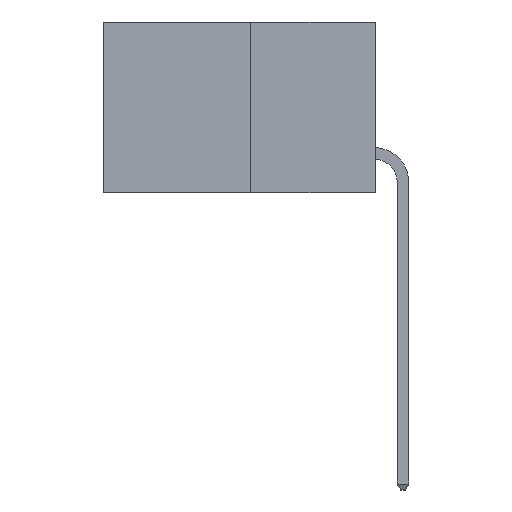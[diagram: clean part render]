
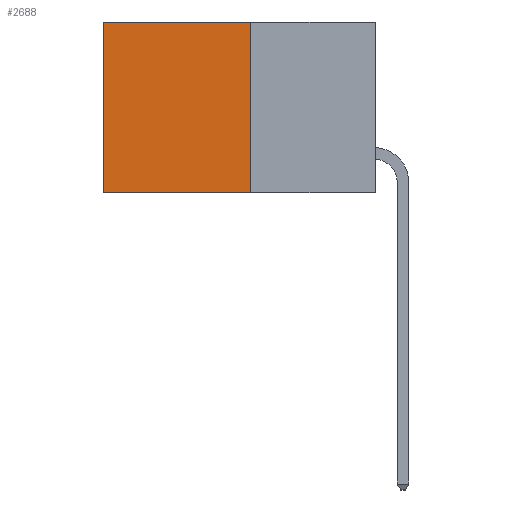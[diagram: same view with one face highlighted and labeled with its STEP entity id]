
A CAD part, left-side view. The second image highlights one B-rep face of the part: STEP entity #2688.
In plain terms, the highlighted planar face has unit normal (-1, 0, 0).
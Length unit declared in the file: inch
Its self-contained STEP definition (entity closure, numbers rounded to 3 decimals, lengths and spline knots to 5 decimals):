
#168 = ORIENTED_EDGE ( 'NONE', *, *, #8321, .T. ) ;
#222 = ORIENTED_EDGE ( 'NONE', *, *, #2465, .F. ) ;
#469 = VERTEX_POINT ( 'NONE', #6813 ) ;
#505 = DIRECTION ( 'NONE',  ( 0., 1., 0. ) ) ;
#796 = DIRECTION ( 'NONE',  ( 0., 1., 0. ) ) ;
#940 = ORIENTED_EDGE ( 'NONE', *, *, #5867, .F. ) ;
#1009 = ORIENTED_EDGE ( 'NONE', *, *, #9448, .T. ) ;
#1093 = VERTEX_POINT ( 'NONE', #1845 ) ;
#1612 = AXIS2_PLACEMENT_3D ( 'NONE', #3009, #3651, #3629 ) ;
#1795 = LINE ( 'NONE', #5422, #3863 ) ;
#1845 = CARTESIAN_POINT ( 'NONE',  ( 0.277, 0.27, -0.37 ) ) ;
#2310 = EDGE_LOOP ( 'NONE', ( #168, #222, #940, #1009 ) ) ;
#2465 = EDGE_CURVE ( 'NONE', #1093, #5009, #3487, .T. ) ;
#2473 = LINE ( 'NONE', #3248, #8045 ) ;
#2688 = ADVANCED_FACE ( 'NONE', ( #8887 ), #2807, .F. ) ;
#2807 = PLANE ( 'NONE',  #1612 ) ;
#3009 = CARTESIAN_POINT ( 'NONE',  ( 0.277, 0.27, -0.37 ) ) ;
#3248 = CARTESIAN_POINT ( 'NONE',  ( 0.277, 0.59, -0.37 ) ) ;
#3319 = VECTOR ( 'NONE', #3657, 39.37008 ) ;
#3486 = CARTESIAN_POINT ( 'NONE',  ( 0.277, 0.27, -0.37 ) ) ;
#3487 = LINE ( 'NONE', #3486, #8995 ) ;
#3629 = DIRECTION ( 'NONE',  ( 0., 0., -1. ) ) ;
#3651 = DIRECTION ( 'NONE',  ( 1., 0., 0. ) ) ;
#3657 = DIRECTION ( 'NONE',  ( 0., 0., -1. ) ) ;
#3663 = CARTESIAN_POINT ( 'NONE',  ( 0.277, 0.27, -0.37 ) ) ;
#3863 = VECTOR ( 'NONE', #796, 39.37008 ) ;
#3970 = VERTEX_POINT ( 'NONE', #7043 ) ;
#4029 = DIRECTION ( 'NONE',  ( 0., 0., -1. ) ) ;
#5009 = VERTEX_POINT ( 'NONE', #8667 ) ;
#5422 = CARTESIAN_POINT ( 'NONE',  ( 0.277, 0.27, 0. ) ) ;
#5867 = EDGE_CURVE ( 'NONE', #3970, #1093, #7430, .T. ) ;
#6813 = CARTESIAN_POINT ( 'NONE',  ( 0.277, 0.59, 0. ) ) ;
#7043 = CARTESIAN_POINT ( 'NONE',  ( 0.277, 0.27, 0. ) ) ;
#7430 = LINE ( 'NONE', #3663, #3319 ) ;
#8045 = VECTOR ( 'NONE', #4029, 39.37008 ) ;
#8321 = EDGE_CURVE ( 'NONE', #469, #5009, #2473, .T. ) ;
#8667 = CARTESIAN_POINT ( 'NONE',  ( 0.277, 0.59, -0.37 ) ) ;
#8887 = FACE_OUTER_BOUND ( 'NONE', #2310, .T. ) ;
#8995 = VECTOR ( 'NONE', #505, 39.37008 ) ;
#9448 = EDGE_CURVE ( 'NONE', #3970, #469, #1795, .T. ) ;
